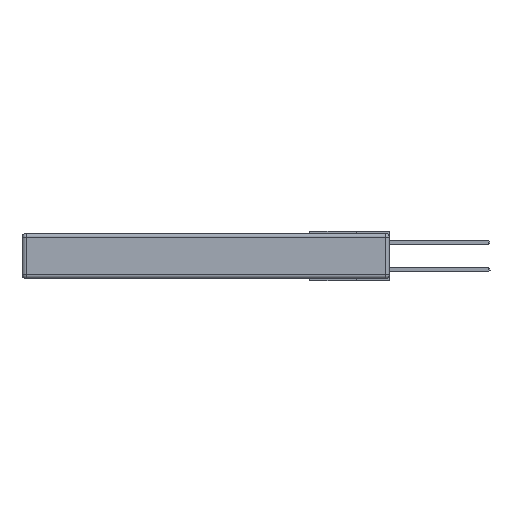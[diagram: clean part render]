
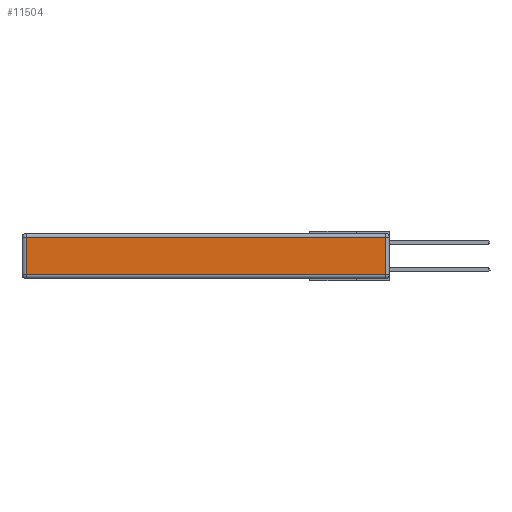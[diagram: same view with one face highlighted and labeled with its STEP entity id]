
A CAD part, left-side view. The second image highlights one B-rep face of the part: STEP entity #11504.
In plain terms, the highlighted planar face has unit normal (-1, 0, 0).
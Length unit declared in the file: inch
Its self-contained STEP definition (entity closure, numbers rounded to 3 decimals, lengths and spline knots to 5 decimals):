
#222 = ORIENTED_EDGE ( 'NONE', *, *, #16578, .T. ) ;
#394 = CARTESIAN_POINT ( 'NONE',  ( 0., 0.03, -0.313 ) ) ;
#613 = LINE ( 'NONE', #9586, #12334 ) ;
#1199 = LINE ( 'NONE', #4715, #15394 ) ;
#1476 = VERTEX_POINT ( 'NONE', #10422 ) ;
#1788 = FACE_OUTER_BOUND ( 'NONE', #1851, .T. ) ;
#1800 = VERTEX_POINT ( 'NONE', #394 ) ;
#1851 = EDGE_LOOP ( 'NONE', ( #10993, #222, #5002, #14362 ) ) ;
#2142 = DIRECTION ( 'NONE',  ( 0., 0., 1. ) ) ;
#2440 = LINE ( 'NONE', #15017, #12503 ) ;
#2700 = PLANE ( 'NONE',  #5663 ) ;
#4078 = CARTESIAN_POINT ( 'NONE',  ( 0., 2.72, -0.03 ) ) ;
#4715 = CARTESIAN_POINT ( 'NONE',  ( 0., 2.75, -0.03 ) ) ;
#4828 = CARTESIAN_POINT ( 'NONE',  ( 0., 2.72, -0.313 ) ) ;
#5002 = ORIENTED_EDGE ( 'NONE', *, *, #10839, .T. ) ;
#5663 = AXIS2_PLACEMENT_3D ( 'NONE', #10453, #9204, #10507 ) ;
#6246 = LINE ( 'NONE', #13804, #10358 ) ;
#6355 = VERTEX_POINT ( 'NONE', #4828 ) ;
#7555 = EDGE_CURVE ( 'NONE', #6355, #1800, #6246, .T. ) ;
#9204 = DIRECTION ( 'NONE',  ( -1., 0., 0. ) ) ;
#9586 = CARTESIAN_POINT ( 'NONE',  ( 0., 2.72, -0.343 ) ) ;
#9618 = EDGE_CURVE ( 'NONE', #14365, #6355, #613, .T. ) ;
#10358 = VECTOR ( 'NONE', #15159, 39.37008 ) ;
#10422 = CARTESIAN_POINT ( 'NONE',  ( 0., 0.03, -0.03 ) ) ;
#10453 = CARTESIAN_POINT ( 'NONE',  ( 0., 0., -0.343 ) ) ;
#10507 = DIRECTION ( 'NONE',  ( 0., 0., 1. ) ) ;
#10839 = EDGE_CURVE ( 'NONE', #1476, #14365, #1199, .T. ) ;
#10993 = ORIENTED_EDGE ( 'NONE', *, *, #7555, .T. ) ;
#11065 = DIRECTION ( 'NONE',  ( 0., 0., -1. ) ) ;
#11504 = ADVANCED_FACE ( 'NONE', ( #1788 ), #2700, .T. ) ;
#12334 = VECTOR ( 'NONE', #11065, 39.37008 ) ;
#12503 = VECTOR ( 'NONE', #2142, 39.37008 ) ;
#13804 = CARTESIAN_POINT ( 'NONE',  ( 0., 0., -0.313 ) ) ;
#13920 = DIRECTION ( 'NONE',  ( 0., 1., 0. ) ) ;
#14362 = ORIENTED_EDGE ( 'NONE', *, *, #9618, .T. ) ;
#14365 = VERTEX_POINT ( 'NONE', #4078 ) ;
#15017 = CARTESIAN_POINT ( 'NONE',  ( 0., 0.03, -0.343 ) ) ;
#15159 = DIRECTION ( 'NONE',  ( 0., -1., 0. ) ) ;
#15394 = VECTOR ( 'NONE', #13920, 39.37008 ) ;
#16578 = EDGE_CURVE ( 'NONE', #1800, #1476, #2440, .T. ) ;
